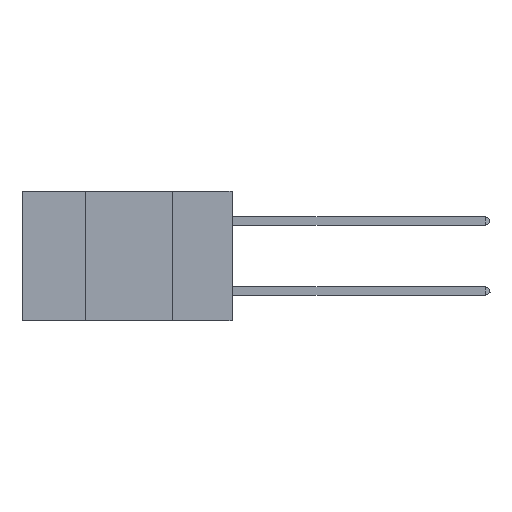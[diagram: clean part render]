
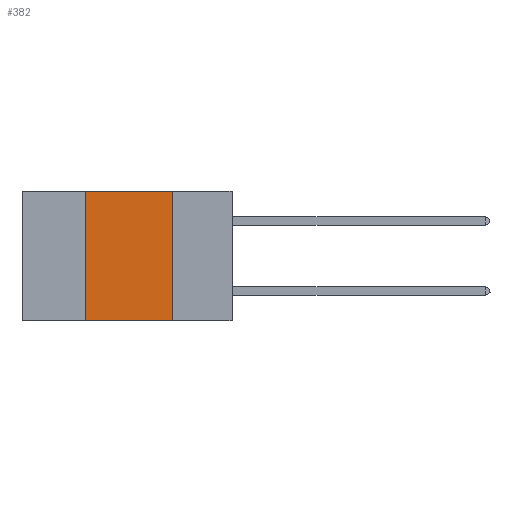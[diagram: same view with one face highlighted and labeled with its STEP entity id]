
A CAD part, left-side view. The second image highlights one B-rep face of the part: STEP entity #382.
In plain terms, the highlighted planar face has unit normal (-1, 0, 0).
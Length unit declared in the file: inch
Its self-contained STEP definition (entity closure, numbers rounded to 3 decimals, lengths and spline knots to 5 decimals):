
#371 = VECTOR ( 'NONE', #11557, 39.37008 ) ;
#382 = ADVANCED_FACE ( 'NONE', ( #11850 ), #8302, .F. ) ;
#394 = CARTESIAN_POINT ( 'NONE',  ( 0., 0.6, -0.37 ) ) ;
#458 = VERTEX_POINT ( 'NONE', #8336 ) ;
#867 = DIRECTION ( 'NONE',  ( 0., 0., -1. ) ) ;
#924 = CARTESIAN_POINT ( 'NONE',  ( 0., 0.17, -0.37 ) ) ;
#2695 = CARTESIAN_POINT ( 'NONE',  ( 0., 0.6, 0. ) ) ;
#3391 = DIRECTION ( 'NONE',  ( 0., 0., 1. ) ) ;
#3505 = ORIENTED_EDGE ( 'NONE', *, *, #8559, .F. ) ;
#3635 = VERTEX_POINT ( 'NONE', #5636 ) ;
#3760 = EDGE_CURVE ( 'NONE', #3635, #458, #6570, .T. ) ;
#4223 = LINE ( 'NONE', #394, #371 ) ;
#5060 = CARTESIAN_POINT ( 'NONE',  ( 0., 0.42, 0. ) ) ;
#5186 = CARTESIAN_POINT ( 'NONE',  ( 0., 0.17, 0. ) ) ;
#5636 = CARTESIAN_POINT ( 'NONE',  ( 0., 0.42, 0. ) ) ;
#5768 = CARTESIAN_POINT ( 'NONE',  ( 0., 0.6, 0. ) ) ;
#6004 = VERTEX_POINT ( 'NONE', #924 ) ;
#6188 = EDGE_LOOP ( 'NONE', ( #3505, #12016, #8331, #11924 ) ) ;
#6570 = LINE ( 'NONE', #5768, #7281 ) ;
#7017 = DIRECTION ( 'NONE',  ( 0., 0., -1. ) ) ;
#7281 = VECTOR ( 'NONE', #8667, 39.37008 ) ;
#7651 = EDGE_CURVE ( 'NONE', #8710, #3635, #8781, .T. ) ;
#8302 = PLANE ( 'NONE',  #9451 ) ;
#8331 = ORIENTED_EDGE ( 'NONE', *, *, #7651, .F. ) ;
#8336 = CARTESIAN_POINT ( 'NONE',  ( 0., 0.17, 0. ) ) ;
#8449 = EDGE_CURVE ( 'NONE', #8710, #6004, #4223, .T. ) ;
#8559 = EDGE_CURVE ( 'NONE', #458, #6004, #9320, .T. ) ;
#8667 = DIRECTION ( 'NONE',  ( 0., -1., 0. ) ) ;
#8710 = VERTEX_POINT ( 'NONE', #10441 ) ;
#8781 = LINE ( 'NONE', #5060, #11590 ) ;
#9320 = LINE ( 'NONE', #5186, #10380 ) ;
#9451 = AXIS2_PLACEMENT_3D ( 'NONE', #2695, #11137, #867 ) ;
#10380 = VECTOR ( 'NONE', #7017, 39.37008 ) ;
#10441 = CARTESIAN_POINT ( 'NONE',  ( 0., 0.42, -0.37 ) ) ;
#11137 = DIRECTION ( 'NONE',  ( 1., 0., 0. ) ) ;
#11557 = DIRECTION ( 'NONE',  ( 0., -1., 0. ) ) ;
#11590 = VECTOR ( 'NONE', #3391, 39.37008 ) ;
#11850 = FACE_OUTER_BOUND ( 'NONE', #6188, .T. ) ;
#11924 = ORIENTED_EDGE ( 'NONE', *, *, #8449, .T. ) ;
#12016 = ORIENTED_EDGE ( 'NONE', *, *, #3760, .F. ) ;
